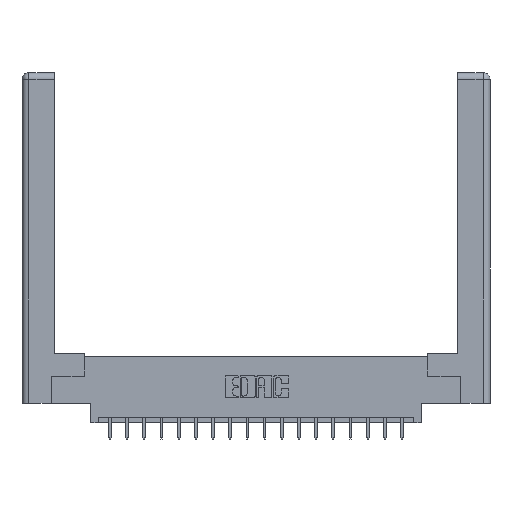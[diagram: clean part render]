
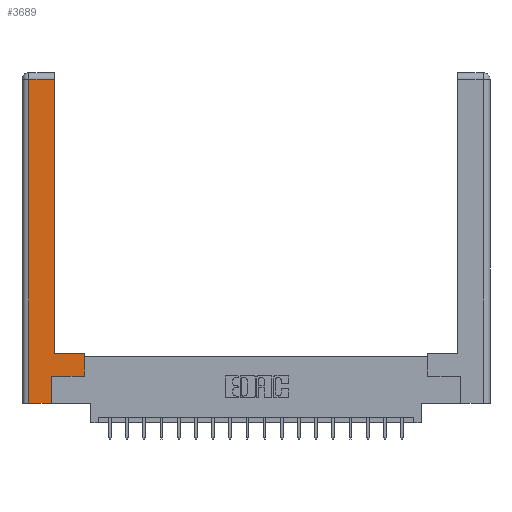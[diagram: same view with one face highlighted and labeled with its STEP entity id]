
A CAD part, top view. The second image highlights one B-rep face of the part: STEP entity #3689.
In plain terms, the highlighted planar face has unit normal (0, 0, 1).
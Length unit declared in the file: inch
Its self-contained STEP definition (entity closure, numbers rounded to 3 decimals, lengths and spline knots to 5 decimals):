
#47 = VECTOR ( 'NONE', #11380, 39.37008 ) ;
#519 = DIRECTION ( 'NONE',  ( -1., 0., 0. ) ) ;
#632 = VERTEX_POINT ( 'NONE', #7387 ) ;
#745 = VECTOR ( 'NONE', #15342, 39.37008 ) ;
#1177 = EDGE_CURVE ( 'NONE', #16945, #632, #11068, .T. ) ;
#1426 = FACE_OUTER_BOUND ( 'NONE', #17492, .T. ) ;
#1745 = VERTEX_POINT ( 'NONE', #7826 ) ;
#1850 = PLANE ( 'NONE',  #16006 ) ;
#2312 = DIRECTION ( 'NONE',  ( 0., 0., -1. ) ) ;
#3689 = ADVANCED_FACE ( 'NONE', ( #1426 ), #1850, .F. ) ;
#3819 = CARTESIAN_POINT ( 'NONE',  ( 0.0615, 2.94, 0. ) ) ;
#3925 = LINE ( 'NONE', #8332, #47 ) ;
#4346 = LINE ( 'NONE', #3819, #6009 ) ;
#4431 = ORIENTED_EDGE ( 'NONE', *, *, #14064, .T. ) ;
#4619 = VECTOR ( 'NONE', #12664, 39.37008 ) ;
#4671 = EDGE_CURVE ( 'NONE', #1745, #6648, #16952, .T. ) ;
#5065 = CARTESIAN_POINT ( 'NONE',  ( 0.0615, 0., 0. ) ) ;
#5222 = CARTESIAN_POINT ( 'NONE',  ( 0.265, 0.245, 0. ) ) ;
#6000 = CARTESIAN_POINT ( 'NONE',  ( 0.295, 2.94, 0. ) ) ;
#6009 = VECTOR ( 'NONE', #519, 39.37008 ) ;
#6046 = VECTOR ( 'NONE', #14899, 39.37008 ) ;
#6470 = EDGE_CURVE ( 'NONE', #17943, #15765, #15658, .T. ) ;
#6628 = EDGE_CURVE ( 'NONE', #6648, #16945, #3925, .T. ) ;
#6648 = VERTEX_POINT ( 'NONE', #6775 ) ;
#6775 = CARTESIAN_POINT ( 'NONE',  ( 0.565, 0.245, 0. ) ) ;
#7341 = VERTEX_POINT ( 'NONE', #6000 ) ;
#7387 = CARTESIAN_POINT ( 'NONE',  ( 0.295, 0.45, 0. ) ) ;
#7826 = CARTESIAN_POINT ( 'NONE',  ( 0.265, 0.245, 0. ) ) ;
#8025 = EDGE_CURVE ( 'NONE', #632, #7341, #12459, .T. ) ;
#8107 = ORIENTED_EDGE ( 'NONE', *, *, #8025, .T. ) ;
#8332 = CARTESIAN_POINT ( 'NONE',  ( 0.565, 0.45, 0. ) ) ;
#8556 = VERTEX_POINT ( 'NONE', #15358 ) ;
#8724 = ORIENTED_EDGE ( 'NONE', *, *, #1177, .T. ) ;
#8754 = CARTESIAN_POINT ( 'NONE',  ( 0.0615, 0., 0. ) ) ;
#8797 = CARTESIAN_POINT ( 'NONE',  ( 0.565, 0.45, 0. ) ) ;
#8883 = DIRECTION ( 'NONE',  ( 0., -1., 0. ) ) ;
#9335 = DIRECTION ( 'NONE',  ( 1., 0., 0. ) ) ;
#9398 = EDGE_CURVE ( 'NONE', #8556, #17943, #19151, .T. ) ;
#9402 = CARTESIAN_POINT ( 'NONE',  ( 0.565, 0.245, 0. ) ) ;
#10430 = LINE ( 'NONE', #5222, #11383 ) ;
#11068 = LINE ( 'NONE', #17959, #6046 ) ;
#11093 = ORIENTED_EDGE ( 'NONE', *, *, #6470, .T. ) ;
#11245 = EDGE_CURVE ( 'NONE', #15765, #1745, #10430, .T. ) ;
#11380 = DIRECTION ( 'NONE',  ( 0., 1., 0. ) ) ;
#11383 = VECTOR ( 'NONE', #17445, 39.37008 ) ;
#11424 = CARTESIAN_POINT ( 'NONE',  ( 0., 0., 0. ) ) ;
#12459 = LINE ( 'NONE', #15140, #745 ) ;
#12508 = ORIENTED_EDGE ( 'NONE', *, *, #6628, .T. ) ;
#12664 = DIRECTION ( 'NONE',  ( 1., 0., 0. ) ) ;
#13921 = CARTESIAN_POINT ( 'NONE',  ( 0.265, 0., 0. ) ) ;
#14064 = EDGE_CURVE ( 'NONE', #7341, #8556, #4346, .T. ) ;
#14141 = ORIENTED_EDGE ( 'NONE', *, *, #9398, .T. ) ;
#14899 = DIRECTION ( 'NONE',  ( -1., 0., 0. ) ) ;
#15140 = CARTESIAN_POINT ( 'NONE',  ( 0.295, 3., 0. ) ) ;
#15342 = DIRECTION ( 'NONE',  ( 0., 1., 0. ) ) ;
#15358 = CARTESIAN_POINT ( 'NONE',  ( 0.0615, 2.94, 0. ) ) ;
#15658 = LINE ( 'NONE', #13921, #4619 ) ;
#15765 = VERTEX_POINT ( 'NONE', #17871 ) ;
#16006 = AXIS2_PLACEMENT_3D ( 'NONE', #11424, #2312, #17497 ) ;
#16337 = ORIENTED_EDGE ( 'NONE', *, *, #4671, .T. ) ;
#16705 = VECTOR ( 'NONE', #9335, 39.37008 ) ;
#16945 = VERTEX_POINT ( 'NONE', #8797 ) ;
#16952 = LINE ( 'NONE', #9402, #16705 ) ;
#17058 = ORIENTED_EDGE ( 'NONE', *, *, #11245, .T. ) ;
#17445 = DIRECTION ( 'NONE',  ( 0., 1., 0. ) ) ;
#17492 = EDGE_LOOP ( 'NONE', ( #8107, #4431, #14141, #11093, #17058, #16337, #12508, #8724 ) ) ;
#17497 = DIRECTION ( 'NONE',  ( -1., 0., 0. ) ) ;
#17732 = VECTOR ( 'NONE', #8883, 39.37008 ) ;
#17871 = CARTESIAN_POINT ( 'NONE',  ( 0.265, 0., 0. ) ) ;
#17943 = VERTEX_POINT ( 'NONE', #5065 ) ;
#17959 = CARTESIAN_POINT ( 'NONE',  ( 0.295, 0.45, 0. ) ) ;
#19151 = LINE ( 'NONE', #8754, #17732 ) ;
